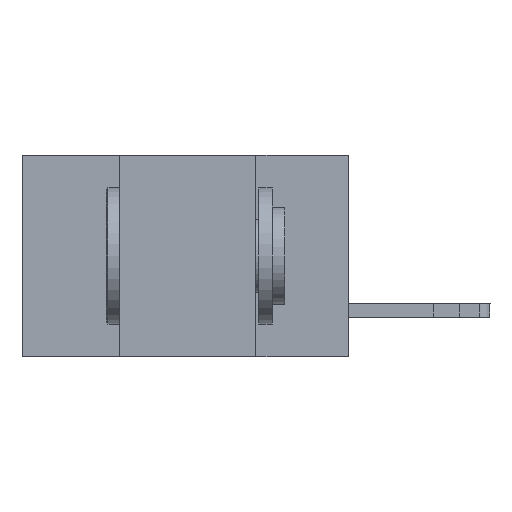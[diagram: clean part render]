
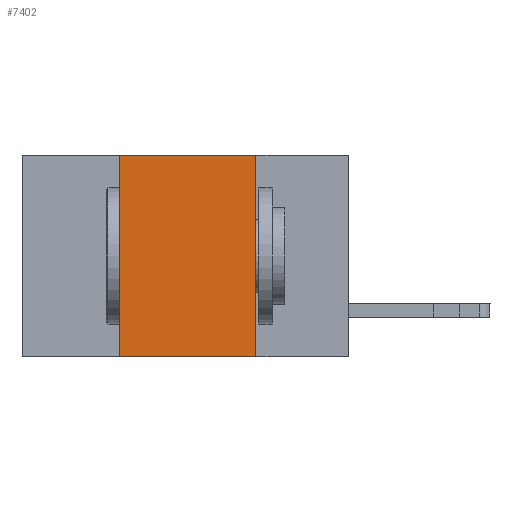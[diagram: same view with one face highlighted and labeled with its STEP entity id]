
A CAD part, left-side view. The second image highlights one B-rep face of the part: STEP entity #7402.
In plain terms, the highlighted planar face has unit normal (-1, 0, 0).
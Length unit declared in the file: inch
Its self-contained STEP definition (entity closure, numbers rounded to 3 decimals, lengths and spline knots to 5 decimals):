
#938 = ORIENTED_EDGE ( 'NONE', *, *, #5366, .F. ) ;
#1072 = CARTESIAN_POINT ( 'NONE',  ( 0., 0.6, -0.37 ) ) ;
#1732 = CARTESIAN_POINT ( 'NONE',  ( 0., 0.17, -0.37 ) ) ;
#1820 = DIRECTION ( 'NONE',  ( 0., 0., -1. ) ) ;
#2423 = VERTEX_POINT ( 'NONE', #17442 ) ;
#3415 = CARTESIAN_POINT ( 'NONE',  ( 0., 0.6, 0. ) ) ;
#5366 = EDGE_CURVE ( 'NONE', #2423, #15806, #6403, .T. ) ;
#5596 = VERTEX_POINT ( 'NONE', #14217 ) ;
#6266 = DIRECTION ( 'NONE',  ( 1., 0., 0. ) ) ;
#6403 = LINE ( 'NONE', #12022, #12513 ) ;
#7152 = EDGE_CURVE ( 'NONE', #16754, #2423, #8138, .T. ) ;
#7312 = VECTOR ( 'NONE', #12310, 39.37008 ) ;
#7402 = ADVANCED_FACE ( 'NONE', ( #16400 ), #10797, .F. ) ;
#7540 = ORIENTED_EDGE ( 'NONE', *, *, #7152, .F. ) ;
#8138 = LINE ( 'NONE', #11280, #15463 ) ;
#8786 = ORIENTED_EDGE ( 'NONE', *, *, #17428, .T. ) ;
#9439 = VECTOR ( 'NONE', #1820, 39.37008 ) ;
#9678 = EDGE_CURVE ( 'NONE', #15806, #5596, #14432, .T. ) ;
#9985 = DIRECTION ( 'NONE',  ( 0., 0., 1. ) ) ;
#10621 = DIRECTION ( 'NONE',  ( 0., 0., -1. ) ) ;
#10797 = PLANE ( 'NONE',  #11925 ) ;
#11162 = ORIENTED_EDGE ( 'NONE', *, *, #9678, .F. ) ;
#11280 = CARTESIAN_POINT ( 'NONE',  ( 0., 0.42, -0.37 ) ) ;
#11842 = CARTESIAN_POINT ( 'NONE',  ( 0., 0.17, 0. ) ) ;
#11925 = AXIS2_PLACEMENT_3D ( 'NONE', #3415, #6266, #10621 ) ;
#11954 = CARTESIAN_POINT ( 'NONE',  ( 0., 0.42, -0.37 ) ) ;
#12022 = CARTESIAN_POINT ( 'NONE',  ( 0., 0.6, 0. ) ) ;
#12310 = DIRECTION ( 'NONE',  ( 0., -1., 0. ) ) ;
#12513 = VECTOR ( 'NONE', #17634, 39.37008 ) ;
#13519 = EDGE_LOOP ( 'NONE', ( #11162, #938, #7540, #8786 ) ) ;
#14217 = CARTESIAN_POINT ( 'NONE',  ( 0., 0.17, -0.37 ) ) ;
#14432 = LINE ( 'NONE', #1732, #9439 ) ;
#15463 = VECTOR ( 'NONE', #9985, 39.37008 ) ;
#15806 = VERTEX_POINT ( 'NONE', #11842 ) ;
#16400 = FACE_OUTER_BOUND ( 'NONE', #13519, .T. ) ;
#16742 = LINE ( 'NONE', #1072, #7312 ) ;
#16754 = VERTEX_POINT ( 'NONE', #11954 ) ;
#17428 = EDGE_CURVE ( 'NONE', #16754, #5596, #16742, .T. ) ;
#17442 = CARTESIAN_POINT ( 'NONE',  ( 0., 0.42, 0. ) ) ;
#17634 = DIRECTION ( 'NONE',  ( 0., -1., 0. ) ) ;
